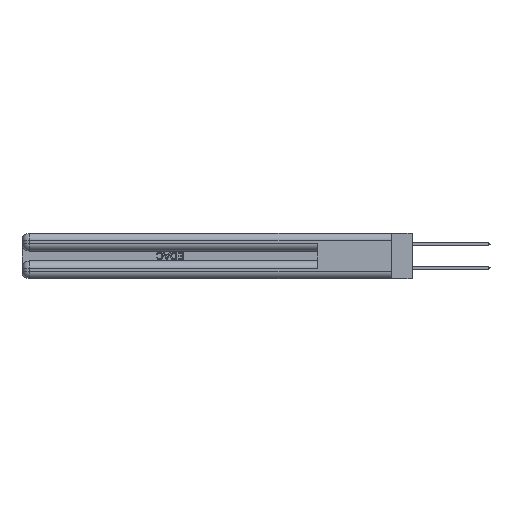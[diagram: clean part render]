
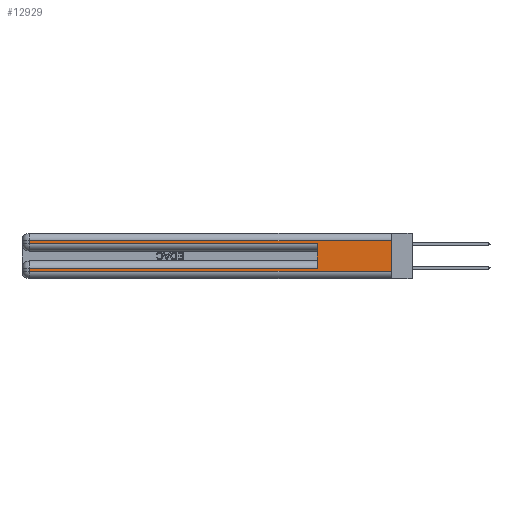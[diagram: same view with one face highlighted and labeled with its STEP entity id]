
A CAD part, left-side view. The second image highlights one B-rep face of the part: STEP entity #12929.
In plain terms, the highlighted planar face has unit normal (-1, 0, 0).
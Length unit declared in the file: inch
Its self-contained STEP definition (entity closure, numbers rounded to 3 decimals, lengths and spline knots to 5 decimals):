
#352 = CARTESIAN_POINT ( 'NONE',  ( 0., 2.94, 0.37 ) ) ;
#635 = FACE_OUTER_BOUND ( 'NONE', #16050, .T. ) ;
#1002 = VERTEX_POINT ( 'NONE', #29025 ) ;
#1286 = CARTESIAN_POINT ( 'NONE',  ( 0., 2.94, 0.285 ) ) ;
#1567 = LINE ( 'NONE', #21898, #10523 ) ;
#1570 = LINE ( 'NONE', #45687, #20564 ) ;
#1841 = PLANE ( 'NONE',  #4418 ) ;
#1998 = DIRECTION ( 'NONE',  ( 1., 0., 0. ) ) ;
#2486 = DIRECTION ( 'NONE',  ( 0., -1., 0. ) ) ;
#2795 = EDGE_CURVE ( 'NONE', #1002, #37004, #1567, .T. ) ;
#3902 = LINE ( 'NONE', #352, #22914 ) ;
#4396 = VERTEX_POINT ( 'NONE', #15842 ) ;
#4418 = AXIS2_PLACEMENT_3D ( 'NONE', #24703, #1998, #28502 ) ;
#5063 = ORIENTED_EDGE ( 'NONE', *, *, #40450, .T. ) ;
#5359 = DIRECTION ( 'NONE',  ( 0., 0., -1. ) ) ;
#5774 = CARTESIAN_POINT ( 'NONE',  ( 0., 0., 0.085 ) ) ;
#6567 = ORIENTED_EDGE ( 'NONE', *, *, #33478, .F. ) ;
#6647 = LINE ( 'NONE', #42913, #16752 ) ;
#6699 = EDGE_CURVE ( 'NONE', #37004, #31963, #3902, .T. ) ;
#7130 = DIRECTION ( 'NONE',  ( 0., 0., -1. ) ) ;
#9618 = DIRECTION ( 'NONE',  ( 0., 1., 0. ) ) ;
#9781 = LINE ( 'NONE', #36355, #47335 ) ;
#10523 = VECTOR ( 'NONE', #25691, 39.37008 ) ;
#10648 = VECTOR ( 'NONE', #7130, 39.37008 ) ;
#11935 = CARTESIAN_POINT ( 'NONE',  ( 0., 2.94, 0.31 ) ) ;
#12544 = ORIENTED_EDGE ( 'NONE', *, *, #2795, .T. ) ;
#12752 = VECTOR ( 'NONE', #9618, 39.37008 ) ;
#12929 = ADVANCED_FACE ( 'NONE', ( #635 ), #1841, .F. ) ;
#13738 = ORIENTED_EDGE ( 'NONE', *, *, #38684, .T. ) ;
#15842 = CARTESIAN_POINT ( 'NONE',  ( 0., 2.94, 0.06 ) ) ;
#16050 = EDGE_LOOP ( 'NONE', ( #6567, #12544, #26438, #42979, #18755, #25736, #13738, #5063 ) ) ;
#16405 = LINE ( 'NONE', #47540, #24063 ) ;
#16752 = VECTOR ( 'NONE', #5359, 39.37008 ) ;
#18755 = ORIENTED_EDGE ( 'NONE', *, *, #44104, .F. ) ;
#19269 = DIRECTION ( 'NONE',  ( 0., 0., -1. ) ) ;
#19371 = VERTEX_POINT ( 'NONE', #33908 ) ;
#20564 = VECTOR ( 'NONE', #41958, 39.37008 ) ;
#21898 = CARTESIAN_POINT ( 'NONE',  ( 0., 0., 0.31 ) ) ;
#22798 = LINE ( 'NONE', #5774, #12752 ) ;
#22914 = VECTOR ( 'NONE', #19269, 39.37008 ) ;
#24063 = VECTOR ( 'NONE', #2486, 39.37008 ) ;
#24703 = CARTESIAN_POINT ( 'NONE',  ( 0., 0., 0.37 ) ) ;
#24872 = VERTEX_POINT ( 'NONE', #26905 ) ;
#24909 = EDGE_CURVE ( 'NONE', #31963, #19371, #1570, .T. ) ;
#25691 = DIRECTION ( 'NONE',  ( 0., 1., 0. ) ) ;
#25736 = ORIENTED_EDGE ( 'NONE', *, *, #26350, .T. ) ;
#26350 = EDGE_CURVE ( 'NONE', #24872, #27994, #22798, .T. ) ;
#26438 = ORIENTED_EDGE ( 'NONE', *, *, #6699, .T. ) ;
#26905 = CARTESIAN_POINT ( 'NONE',  ( 0., 0.6, 0.085 ) ) ;
#27994 = VERTEX_POINT ( 'NONE', #41610 ) ;
#28502 = DIRECTION ( 'NONE',  ( 0., 0., -1. ) ) ;
#29025 = CARTESIAN_POINT ( 'NONE',  ( 0., 0., 0.31 ) ) ;
#31963 = VERTEX_POINT ( 'NONE', #1286 ) ;
#33478 = EDGE_CURVE ( 'NONE', #1002, #45952, #6647, .T. ) ;
#33908 = CARTESIAN_POINT ( 'NONE',  ( 0., 0.6, 0.285 ) ) ;
#34260 = CARTESIAN_POINT ( 'NONE',  ( 0., 0., 0.06 ) ) ;
#36355 = CARTESIAN_POINT ( 'NONE',  ( 0., 0.6, 0.145 ) ) ;
#37004 = VERTEX_POINT ( 'NONE', #11935 ) ;
#38684 = EDGE_CURVE ( 'NONE', #27994, #4396, #41803, .T. ) ;
#40112 = DIRECTION ( 'NONE',  ( 0., 0., 1. ) ) ;
#40450 = EDGE_CURVE ( 'NONE', #4396, #45952, #16405, .T. ) ;
#41610 = CARTESIAN_POINT ( 'NONE',  ( 0., 2.94, 0.085 ) ) ;
#41803 = LINE ( 'NONE', #44633, #10648 ) ;
#41958 = DIRECTION ( 'NONE',  ( 0., -1., 0. ) ) ;
#42913 = CARTESIAN_POINT ( 'NONE',  ( 0., 0., 0.37 ) ) ;
#42979 = ORIENTED_EDGE ( 'NONE', *, *, #24909, .T. ) ;
#44104 = EDGE_CURVE ( 'NONE', #24872, #19371, #9781, .T. ) ;
#44633 = CARTESIAN_POINT ( 'NONE',  ( 0., 2.94, 0.37 ) ) ;
#45687 = CARTESIAN_POINT ( 'NONE',  ( 0., 0., 0.285 ) ) ;
#45952 = VERTEX_POINT ( 'NONE', #34260 ) ;
#47335 = VECTOR ( 'NONE', #40112, 39.37008 ) ;
#47540 = CARTESIAN_POINT ( 'NONE',  ( 0., 0., 0.06 ) ) ;
